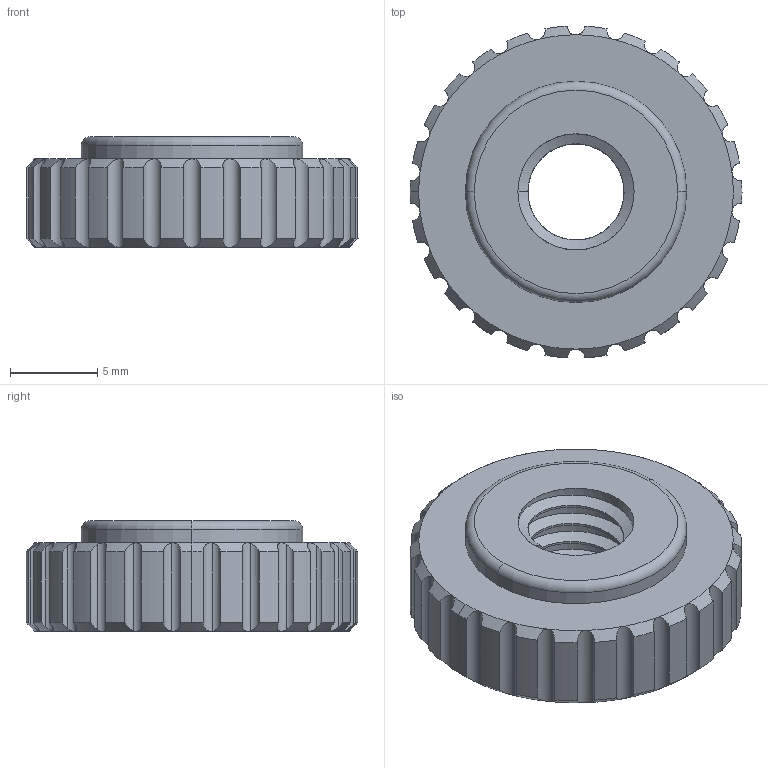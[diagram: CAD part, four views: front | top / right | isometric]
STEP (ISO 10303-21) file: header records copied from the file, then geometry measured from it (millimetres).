
FILE_DESCRIPTION (( 'STEP AP203' ), '1' );
FILE_NAME ('AF-WF-GS-PRT-005-STEP.STEP', '2020-07-21T18:58:06', ( '' ), ( '' ), 'SwSTEP 2.0', 'SolidWorks 2018', '' );
FILE_SCHEMA (( 'CONFIG_CONTROL_DESIGN' ));
Length unit declared in the file: inch
Products named in the file (1): AF-WF-GS-PRT-005-STEP
Bounding box: 19.05 x 19.02 x 6.35 mm (x, y, z)
Volume: 1347.3 mm3; surface area: 1054 mm2
Topology: 1 solids, 1 shells, 141 faces, 355 edges, 217 vertices
Faces by surface type: cylinder 78, cone 54, plane 4, bspline 3, torus 2
Entity records: 5623 total; most frequent: CARTESIAN_POINT 2414, ORIENTED_EDGE 710, DIRECTION 601, EDGE_CURVE 355, AXIS2_PLACEMENT_3D 259, VERTEX_POINT 217, EDGE_LOOP 144, FACE_OUTER_BOUND 141
